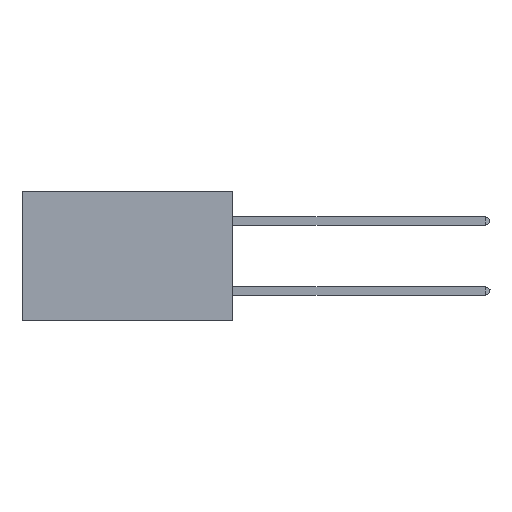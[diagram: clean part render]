
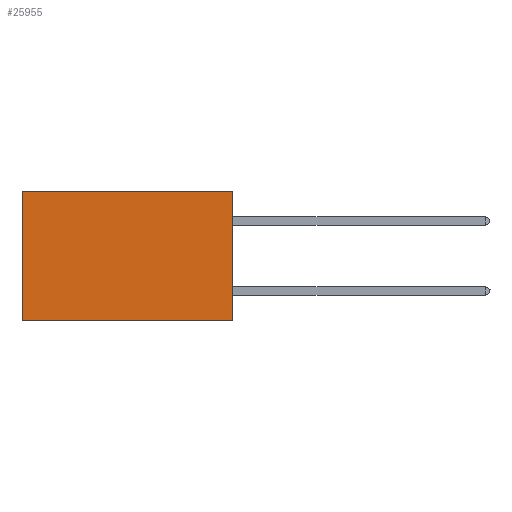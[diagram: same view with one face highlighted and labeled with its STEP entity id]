
A CAD part, left-side view. The second image highlights one B-rep face of the part: STEP entity #25955.
In plain terms, the highlighted planar face has unit normal (-1, 0, 0).
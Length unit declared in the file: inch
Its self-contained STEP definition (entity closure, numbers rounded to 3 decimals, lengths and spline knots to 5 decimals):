
#2964 = CARTESIAN_POINT ( 'NONE',  ( 0.2875, 0., 0. ) ) ;
#3473 = VECTOR ( 'NONE', #12808, 39.37008 ) ;
#3649 = PLANE ( 'NONE',  #21533 ) ;
#3841 = VERTEX_POINT ( 'NONE', #24888 ) ;
#4251 = LINE ( 'NONE', #12497, #9983 ) ;
#4659 = DIRECTION ( 'NONE',  ( 0., 1., 0. ) ) ;
#5014 = VECTOR ( 'NONE', #12539, 39.37008 ) ;
#6236 = EDGE_CURVE ( 'NONE', #3841, #28768, #17667, .T. ) ;
#9983 = VECTOR ( 'NONE', #32079, 39.37008 ) ;
#12497 = CARTESIAN_POINT ( 'NONE',  ( 0.2875, 0.6, 0. ) ) ;
#12539 = DIRECTION ( 'NONE',  ( 0., 0., -1. ) ) ;
#12634 = CARTESIAN_POINT ( 'NONE',  ( 0.2875, 0.6, 0. ) ) ;
#12808 = DIRECTION ( 'NONE',  ( 0., 1., 0. ) ) ;
#12864 = EDGE_CURVE ( 'NONE', #34800, #28566, #29582, .T. ) ;
#13702 = VECTOR ( 'NONE', #4659, 39.37008 ) ;
#14565 = CARTESIAN_POINT ( 'NONE',  ( 0.2875, 0., 0. ) ) ;
#17435 = EDGE_LOOP ( 'NONE', ( #32485, #33857, #22495, #22754 ) ) ;
#17667 = LINE ( 'NONE', #24495, #13702 ) ;
#20283 = FACE_OUTER_BOUND ( 'NONE', #17435, .T. ) ;
#21533 = AXIS2_PLACEMENT_3D ( 'NONE', #14565, #23455, #26190 ) ;
#22495 = ORIENTED_EDGE ( 'NONE', *, *, #33770, .F. ) ;
#22754 = ORIENTED_EDGE ( 'NONE', *, *, #12864, .T. ) ;
#23455 = DIRECTION ( 'NONE',  ( 1., 0., 0. ) ) ;
#24495 = CARTESIAN_POINT ( 'NONE',  ( 0.2875, 0., -0.37 ) ) ;
#24505 = LINE ( 'NONE', #29497, #5014 ) ;
#24888 = CARTESIAN_POINT ( 'NONE',  ( 0.2875, 0., -0.37 ) ) ;
#25955 = ADVANCED_FACE ( 'NONE', ( #20283 ), #3649, .F. ) ;
#26190 = DIRECTION ( 'NONE',  ( 0., 0., -1. ) ) ;
#26565 = CARTESIAN_POINT ( 'NONE',  ( 0.2875, 0., 0. ) ) ;
#28566 = VERTEX_POINT ( 'NONE', #12634 ) ;
#28768 = VERTEX_POINT ( 'NONE', #32706 ) ;
#29497 = CARTESIAN_POINT ( 'NONE',  ( 0.2875, 0., 0. ) ) ;
#29582 = LINE ( 'NONE', #26565, #3473 ) ;
#32079 = DIRECTION ( 'NONE',  ( 0., 0., -1. ) ) ;
#32221 = EDGE_CURVE ( 'NONE', #28566, #28768, #4251, .T. ) ;
#32485 = ORIENTED_EDGE ( 'NONE', *, *, #32221, .T. ) ;
#32706 = CARTESIAN_POINT ( 'NONE',  ( 0.2875, 0.6, -0.37 ) ) ;
#33770 = EDGE_CURVE ( 'NONE', #34800, #3841, #24505, .T. ) ;
#33857 = ORIENTED_EDGE ( 'NONE', *, *, #6236, .F. ) ;
#34800 = VERTEX_POINT ( 'NONE', #2964 ) ;
